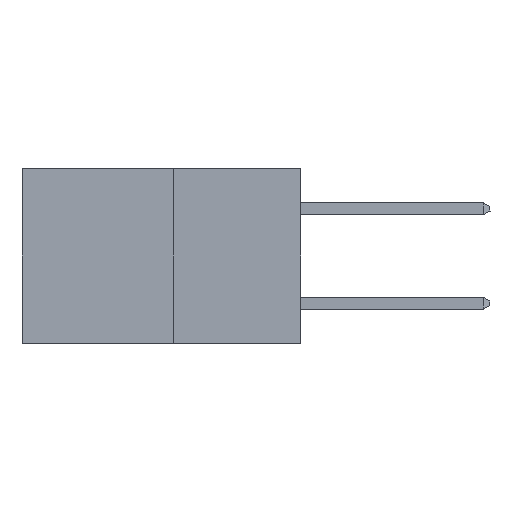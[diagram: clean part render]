
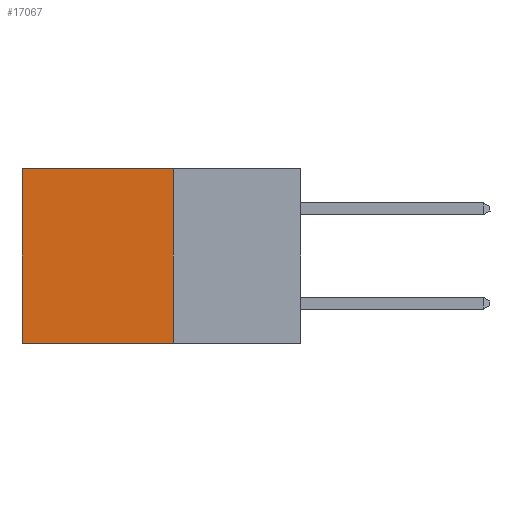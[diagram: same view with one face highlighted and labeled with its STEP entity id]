
A CAD part, left-side view. The second image highlights one B-rep face of the part: STEP entity #17067.
In plain terms, the highlighted planar face has unit normal (-1, 0, 0).
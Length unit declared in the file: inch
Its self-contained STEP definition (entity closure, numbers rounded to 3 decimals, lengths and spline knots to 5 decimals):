
#89 = EDGE_LOOP ( 'NONE', ( #6575, #20298, #15429, #4219 ) ) ;
#835 = CARTESIAN_POINT ( 'NONE',  ( 0.277, 0.27, -0.37 ) ) ;
#2093 = VECTOR ( 'NONE', #13354, 39.37008 ) ;
#2667 = EDGE_CURVE ( 'NONE', #20827, #17520, #15120, .T. ) ;
#3007 = CARTESIAN_POINT ( 'NONE',  ( 0.277, 0.59, 0. ) ) ;
#3079 = PLANE ( 'NONE',  #16259 ) ;
#3249 = CARTESIAN_POINT ( 'NONE',  ( 0.277, 0.27, 0. ) ) ;
#3855 = CARTESIAN_POINT ( 'NONE',  ( 0.277, 0.59, -0.37 ) ) ;
#4219 = ORIENTED_EDGE ( 'NONE', *, *, #16443, .T. ) ;
#4864 = DIRECTION ( 'NONE',  ( 0., 1., 0. ) ) ;
#5922 = EDGE_CURVE ( 'NONE', #17038, #20212, #15240, .T. ) ;
#6389 = DIRECTION ( 'NONE',  ( 0., 0., -1. ) ) ;
#6575 = ORIENTED_EDGE ( 'NONE', *, *, #5922, .T. ) ;
#6840 = VECTOR ( 'NONE', #4864, 39.37008 ) ;
#7430 = EDGE_CURVE ( 'NONE', #17520, #20212, #15934, .T. ) ;
#7662 = CARTESIAN_POINT ( 'NONE',  ( 0.277, 0.27, -0.37 ) ) ;
#10676 = DIRECTION ( 'NONE',  ( 0., 1., 0. ) ) ;
#11199 = LINE ( 'NONE', #3249, #6840 ) ;
#11654 = VECTOR ( 'NONE', #10676, 39.37008 ) ;
#13354 = DIRECTION ( 'NONE',  ( 0., 0., -1. ) ) ;
#14515 = CARTESIAN_POINT ( 'NONE',  ( 0.277, 0.27, -0.37 ) ) ;
#15120 = LINE ( 'NONE', #15167, #2093 ) ;
#15167 = CARTESIAN_POINT ( 'NONE',  ( 0.277, 0.27, -0.37 ) ) ;
#15240 = LINE ( 'NONE', #18124, #18985 ) ;
#15429 = ORIENTED_EDGE ( 'NONE', *, *, #2667, .F. ) ;
#15934 = LINE ( 'NONE', #835, #11654 ) ;
#16150 = DIRECTION ( 'NONE',  ( 1., 0., 0. ) ) ;
#16259 = AXIS2_PLACEMENT_3D ( 'NONE', #14515, #16150, #6389 ) ;
#16443 = EDGE_CURVE ( 'NONE', #20827, #17038, #11199, .T. ) ;
#16532 = DIRECTION ( 'NONE',  ( 0., 0., -1. ) ) ;
#16731 = FACE_OUTER_BOUND ( 'NONE', #89, .T. ) ;
#17038 = VERTEX_POINT ( 'NONE', #3007 ) ;
#17067 = ADVANCED_FACE ( 'NONE', ( #16731 ), #3079, .F. ) ;
#17520 = VERTEX_POINT ( 'NONE', #7662 ) ;
#18124 = CARTESIAN_POINT ( 'NONE',  ( 0.277, 0.59, -0.37 ) ) ;
#18254 = CARTESIAN_POINT ( 'NONE',  ( 0.277, 0.27, 0. ) ) ;
#18985 = VECTOR ( 'NONE', #16532, 39.37008 ) ;
#20212 = VERTEX_POINT ( 'NONE', #3855 ) ;
#20298 = ORIENTED_EDGE ( 'NONE', *, *, #7430, .F. ) ;
#20827 = VERTEX_POINT ( 'NONE', #18254 ) ;
